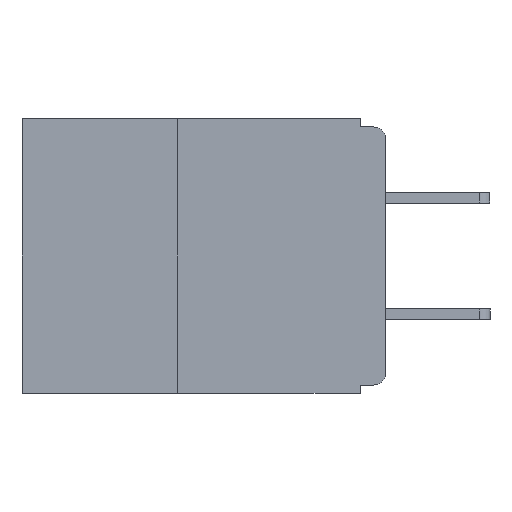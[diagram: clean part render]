
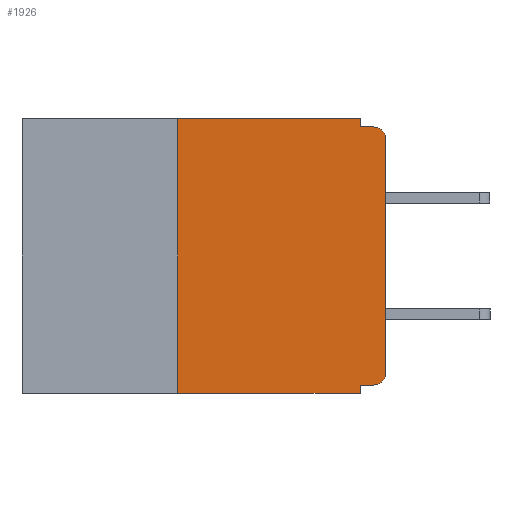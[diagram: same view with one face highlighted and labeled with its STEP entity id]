
A CAD part, left-side view. The second image highlights one B-rep face of the part: STEP entity #1926.
In plain terms, the highlighted planar face has unit normal (-1, 0, 0).
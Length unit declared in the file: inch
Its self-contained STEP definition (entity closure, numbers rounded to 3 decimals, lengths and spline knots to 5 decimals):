
#391 = CARTESIAN_POINT ( 'NONE',  ( 0., 0.031, -0.32 ) ) ;
#681 = VERTEX_POINT ( 'NONE', #3603 ) ;
#746 = CARTESIAN_POINT ( 'NONE',  ( 0., 0., -0.32 ) ) ;
#1118 = VECTOR ( 'NONE', #10346, 39.37008 ) ;
#1623 = EDGE_CURVE ( 'NONE', #14378, #15614, #17891, .T. ) ;
#1625 = DIRECTION ( 'NONE',  ( -1., 0., 0. ) ) ;
#1926 = ADVANCED_FACE ( 'NONE', ( #16727 ), #18346, .F. ) ;
#1989 = ORIENTED_EDGE ( 'NONE', *, *, #2273, .F. ) ;
#2273 = EDGE_CURVE ( 'NONE', #7810, #15614, #25389, .T. ) ;
#2675 = DIRECTION ( 'NONE',  ( 0., 0., -1. ) ) ;
#2994 = DIRECTION ( 'NONE',  ( -1., 0., 0. ) ) ;
#3086 = VECTOR ( 'NONE', #20647, 39.37008 ) ;
#3464 = CARTESIAN_POINT ( 'NONE',  ( 0., 0.031, -0.33 ) ) ;
#3603 = CARTESIAN_POINT ( 'NONE',  ( 0., 0.031, 0. ) ) ;
#3851 = AXIS2_PLACEMENT_3D ( 'NONE', #24525, #2994, #2675 ) ;
#3947 = CARTESIAN_POINT ( 'NONE',  ( 0., 0.437, -0.33 ) ) ;
#4293 = LINE ( 'NONE', #30807, #29372 ) ;
#4809 = CARTESIAN_POINT ( 'NONE',  ( 0., 0., -0.305 ) ) ;
#5220 = CARTESIAN_POINT ( 'NONE',  ( 0., 0., -0.01 ) ) ;
#5467 = CARTESIAN_POINT ( 'NONE',  ( 0., 0.25, -0.33 ) ) ;
#6416 = DIRECTION ( 'NONE',  ( 0., -1., 0. ) ) ;
#6519 = VERTEX_POINT ( 'NONE', #391 ) ;
#6594 = LINE ( 'NONE', #11444, #30093 ) ;
#6783 = ORIENTED_EDGE ( 'NONE', *, *, #25244, .F. ) ;
#7000 = VERTEX_POINT ( 'NONE', #23806 ) ;
#7267 = EDGE_CURVE ( 'NONE', #681, #7810, #6594, .T. ) ;
#7810 = VERTEX_POINT ( 'NONE', #15079 ) ;
#7873 = EDGE_CURVE ( 'NONE', #26357, #14378, #14306, .T. ) ;
#8204 = ORIENTED_EDGE ( 'NONE', *, *, #7267, .F. ) ;
#8243 = CARTESIAN_POINT ( 'NONE',  ( 0., 0., -0.025 ) ) ;
#8604 = CARTESIAN_POINT ( 'NONE',  ( 0., 0.015, -0.01 ) ) ;
#8837 = VERTEX_POINT ( 'NONE', #26173 ) ;
#9670 = VECTOR ( 'NONE', #13120, 39.37008 ) ;
#10346 = DIRECTION ( 'NONE',  ( 0., 0., 1. ) ) ;
#10720 = DIRECTION ( 'NONE',  ( 0., 0., -1. ) ) ;
#11375 = VERTEX_POINT ( 'NONE', #5467 ) ;
#11444 = CARTESIAN_POINT ( 'NONE',  ( 0., 0.031, 0. ) ) ;
#11655 = EDGE_CURVE ( 'NONE', #22313, #26357, #22849, .T. ) ;
#12837 = CARTESIAN_POINT ( 'NONE',  ( 0., 0., 0. ) ) ;
#12905 = ORIENTED_EDGE ( 'NONE', *, *, #13945, .F. ) ;
#13120 = DIRECTION ( 'NONE',  ( 0., 1., 0. ) ) ;
#13945 = EDGE_CURVE ( 'NONE', #11375, #7000, #4293, .T. ) ;
#14306 = LINE ( 'NONE', #12837, #1118 ) ;
#14378 = VERTEX_POINT ( 'NONE', #8243 ) ;
#15079 = CARTESIAN_POINT ( 'NONE',  ( 0., 0.031, -0.01 ) ) ;
#15567 = ORIENTED_EDGE ( 'NONE', *, *, #1623, .T. ) ;
#15614 = VERTEX_POINT ( 'NONE', #8604 ) ;
#15635 = DIRECTION ( 'NONE',  ( 1., 0., 0. ) ) ;
#15643 = DIRECTION ( 'NONE',  ( 0., 0., -1. ) ) ;
#16439 = CARTESIAN_POINT ( 'NONE',  ( 0., 0.015, -0.305 ) ) ;
#16531 = DIRECTION ( 'NONE',  ( 0., 0., 1. ) ) ;
#16727 = FACE_OUTER_BOUND ( 'NONE', #21444, .T. ) ;
#16965 = LINE ( 'NONE', #746, #9670 ) ;
#17143 = EDGE_CURVE ( 'NONE', #7000, #681, #29181, .T. ) ;
#17623 = ORIENTED_EDGE ( 'NONE', *, *, #18799, .T. ) ;
#17891 = CIRCLE ( 'NONE', #3851, 0.015 ) ;
#18260 = LINE ( 'NONE', #3947, #30211 ) ;
#18346 = PLANE ( 'NONE',  #28307 ) ;
#18799 = EDGE_CURVE ( 'NONE', #11375, #8837, #18260, .T. ) ;
#18861 = DIRECTION ( 'NONE',  ( 0., 0., -1. ) ) ;
#19617 = DIRECTION ( 'NONE',  ( 0., -1., 0. ) ) ;
#19726 = VECTOR ( 'NONE', #23262, 39.37008 ) ;
#20647 = DIRECTION ( 'NONE',  ( 0., 0., -1. ) ) ;
#21133 = LINE ( 'NONE', #3464, #3086 ) ;
#21444 = EDGE_LOOP ( 'NONE', ( #29770, #15567, #1989, #8204, #25720, #12905, #17623, #21711, #6783, #31122 ) ) ;
#21711 = ORIENTED_EDGE ( 'NONE', *, *, #25290, .F. ) ;
#22118 = VECTOR ( 'NONE', #19617, 39.37008 ) ;
#22313 = VERTEX_POINT ( 'NONE', #24730 ) ;
#22849 = CIRCLE ( 'NONE', #24335, 0.015 ) ;
#23262 = DIRECTION ( 'NONE',  ( 0., -1., 0. ) ) ;
#23806 = CARTESIAN_POINT ( 'NONE',  ( 0., 0.25, 0. ) ) ;
#24335 = AXIS2_PLACEMENT_3D ( 'NONE', #16439, #1625, #18861 ) ;
#24525 = CARTESIAN_POINT ( 'NONE',  ( 0., 0.015, -0.025 ) ) ;
#24730 = CARTESIAN_POINT ( 'NONE',  ( 0., 0.015, -0.32 ) ) ;
#25244 = EDGE_CURVE ( 'NONE', #22313, #6519, #16965, .T. ) ;
#25290 = EDGE_CURVE ( 'NONE', #6519, #8837, #21133, .T. ) ;
#25389 = LINE ( 'NONE', #5220, #19726 ) ;
#25720 = ORIENTED_EDGE ( 'NONE', *, *, #17143, .F. ) ;
#26173 = CARTESIAN_POINT ( 'NONE',  ( 0., 0.031, -0.33 ) ) ;
#26357 = VERTEX_POINT ( 'NONE', #4809 ) ;
#28307 = AXIS2_PLACEMENT_3D ( 'NONE', #29298, #15635, #15643 ) ;
#29181 = LINE ( 'NONE', #31413, #22118 ) ;
#29298 = CARTESIAN_POINT ( 'NONE',  ( 0., 0.437, 0. ) ) ;
#29372 = VECTOR ( 'NONE', #16531, 39.37008 ) ;
#29770 = ORIENTED_EDGE ( 'NONE', *, *, #7873, .T. ) ;
#30093 = VECTOR ( 'NONE', #10720, 39.37008 ) ;
#30211 = VECTOR ( 'NONE', #6416, 39.37008 ) ;
#30807 = CARTESIAN_POINT ( 'NONE',  ( 0., 0.25, -0.33 ) ) ;
#31122 = ORIENTED_EDGE ( 'NONE', *, *, #11655, .T. ) ;
#31413 = CARTESIAN_POINT ( 'NONE',  ( 0., 0.437, 0. ) ) ;
